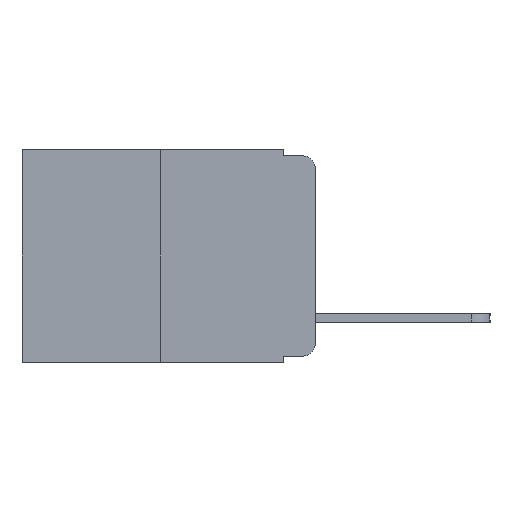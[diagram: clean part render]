
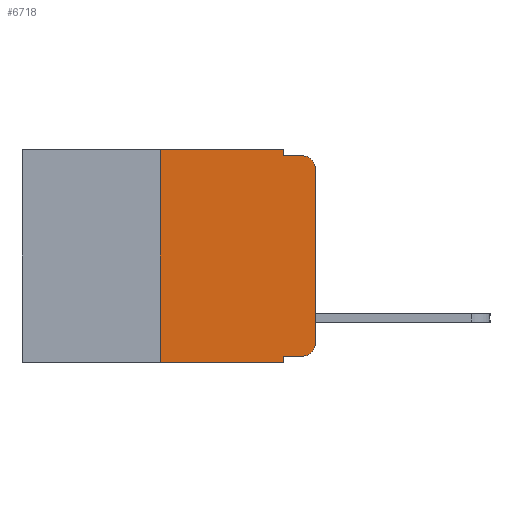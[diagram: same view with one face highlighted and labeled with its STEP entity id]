
A CAD part, left-side view. The second image highlights one B-rep face of the part: STEP entity #6718.
In plain terms, the highlighted planar face has unit normal (-1, 0, 0).
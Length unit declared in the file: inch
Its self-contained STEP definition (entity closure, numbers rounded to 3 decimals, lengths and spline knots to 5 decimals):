
#108 = EDGE_CURVE ( 'NONE', #347, #9766, #10966, .T. ) ;
#344 = LINE ( 'NONE', #10707, #2691 ) ;
#347 = VERTEX_POINT ( 'NONE', #3068 ) ;
#433 = ORIENTED_EDGE ( 'NONE', *, *, #10182, .T. ) ;
#492 = LINE ( 'NONE', #6207, #7602 ) ;
#597 = CARTESIAN_POINT ( 'NONE',  ( 0., 0.051, -0.343 ) ) ;
#741 = ORIENTED_EDGE ( 'NONE', *, *, #4778, .F. ) ;
#763 = VERTEX_POINT ( 'NONE', #1456 ) ;
#1041 = EDGE_LOOP ( 'NONE', ( #3531, #6307, #741, #2929, #4317, #3243, #433, #4896, #4964, #11048 ) ) ;
#1456 = CARTESIAN_POINT ( 'NONE',  ( 0., 0.25, 0. ) ) ;
#1543 = EDGE_CURVE ( 'NONE', #8922, #763, #7137, .T. ) ;
#1604 = VECTOR ( 'NONE', #5992, 39.37008 ) ;
#1608 = EDGE_CURVE ( 'NONE', #6167, #1844, #5993, .T. ) ;
#1651 = EDGE_CURVE ( 'NONE', #6167, #8879, #492, .T. ) ;
#1710 = EDGE_CURVE ( 'NONE', #8879, #10385, #4949, .T. ) ;
#1844 = VERTEX_POINT ( 'NONE', #597 ) ;
#1911 = CARTESIAN_POINT ( 'NONE',  ( 0., 0.473, 0. ) ) ;
#2230 = VECTOR ( 'NONE', #9896, 39.37008 ) ;
#2691 = VECTOR ( 'NONE', #4604, 39.37008 ) ;
#2699 = DIRECTION ( 'NONE',  ( 0., 0., 1. ) ) ;
#2929 = ORIENTED_EDGE ( 'NONE', *, *, #108, .F. ) ;
#3068 = CARTESIAN_POINT ( 'NONE',  ( 0., 0.051, 0. ) ) ;
#3088 = VECTOR ( 'NONE', #8854, 39.37008 ) ;
#3243 = ORIENTED_EDGE ( 'NONE', *, *, #1543, .F. ) ;
#3495 = LINE ( 'NONE', #4232, #5549 ) ;
#3531 = ORIENTED_EDGE ( 'NONE', *, *, #3992, .T. ) ;
#3609 = VERTEX_POINT ( 'NONE', #5824 ) ;
#3943 = DIRECTION ( 'NONE',  ( -1., 0., 0. ) ) ;
#3964 = CARTESIAN_POINT ( 'NONE',  ( 0., 0.02, -0.313 ) ) ;
#3992 = EDGE_CURVE ( 'NONE', #10385, #3609, #6940, .T. ) ;
#4232 = CARTESIAN_POINT ( 'NONE',  ( 0., 0.051, -0.01 ) ) ;
#4317 = ORIENTED_EDGE ( 'NONE', *, *, #7334, .F. ) ;
#4354 = CARTESIAN_POINT ( 'NONE',  ( 0., 0.051, 0. ) ) ;
#4382 = EDGE_CURVE ( 'NONE', #3609, #9949, #10866, .T. ) ;
#4604 = DIRECTION ( 'NONE',  ( 0., -1., 0. ) ) ;
#4610 = DIRECTION ( 'NONE',  ( -1., 0., 0. ) ) ;
#4635 = CARTESIAN_POINT ( 'NONE',  ( 0., 0.02, -0.03 ) ) ;
#4778 = EDGE_CURVE ( 'NONE', #9766, #9949, #3495, .T. ) ;
#4896 = ORIENTED_EDGE ( 'NONE', *, *, #1608, .F. ) ;
#4949 = CIRCLE ( 'NONE', #5562, 0.02 ) ;
#4964 = ORIENTED_EDGE ( 'NONE', *, *, #1651, .T. ) ;
#5166 = CARTESIAN_POINT ( 'NONE',  ( 0., 0.25, 0. ) ) ;
#5179 = CARTESIAN_POINT ( 'NONE',  ( 0., 0.02, -0.01 ) ) ;
#5362 = DIRECTION ( 'NONE',  ( 0., 0., -1. ) ) ;
#5549 = VECTOR ( 'NONE', #6729, 39.37008 ) ;
#5562 = AXIS2_PLACEMENT_3D ( 'NONE', #3964, #3943, #10458 ) ;
#5824 = CARTESIAN_POINT ( 'NONE',  ( 0., 0., -0.03 ) ) ;
#5992 = DIRECTION ( 'NONE',  ( 0., 0., -1. ) ) ;
#5993 = LINE ( 'NONE', #10752, #10439 ) ;
#6052 = CARTESIAN_POINT ( 'NONE',  ( 0., 0.473, 0. ) ) ;
#6167 = VERTEX_POINT ( 'NONE', #8974 ) ;
#6207 = CARTESIAN_POINT ( 'NONE',  ( 0., 0.051, -0.333 ) ) ;
#6307 = ORIENTED_EDGE ( 'NONE', *, *, #4382, .T. ) ;
#6631 = CARTESIAN_POINT ( 'NONE',  ( 0., 0., -0.313 ) ) ;
#6718 = ADVANCED_FACE ( 'NONE', ( #9049 ), #11382, .F. ) ;
#6729 = DIRECTION ( 'NONE',  ( 0., -1., 0. ) ) ;
#6940 = LINE ( 'NONE', #9470, #2230 ) ;
#7137 = LINE ( 'NONE', #5166, #9520 ) ;
#7334 = EDGE_CURVE ( 'NONE', #763, #347, #7851, .T. ) ;
#7416 = CARTESIAN_POINT ( 'NONE',  ( 0., 0.02, -0.333 ) ) ;
#7602 = VECTOR ( 'NONE', #10845, 39.37008 ) ;
#7660 = CARTESIAN_POINT ( 'NONE',  ( 0., 0.051, -0.01 ) ) ;
#7716 = AXIS2_PLACEMENT_3D ( 'NONE', #4635, #4610, #5362 ) ;
#7851 = LINE ( 'NONE', #1911, #3088 ) ;
#8854 = DIRECTION ( 'NONE',  ( 0., -1., 0. ) ) ;
#8879 = VERTEX_POINT ( 'NONE', #7416 ) ;
#8922 = VERTEX_POINT ( 'NONE', #11595 ) ;
#8974 = CARTESIAN_POINT ( 'NONE',  ( 0., 0.051, -0.333 ) ) ;
#9049 = FACE_OUTER_BOUND ( 'NONE', #1041, .T. ) ;
#9470 = CARTESIAN_POINT ( 'NONE',  ( 0., 0., 0. ) ) ;
#9520 = VECTOR ( 'NONE', #2699, 39.37008 ) ;
#9766 = VERTEX_POINT ( 'NONE', #7660 ) ;
#9896 = DIRECTION ( 'NONE',  ( 0., 0., 1. ) ) ;
#9949 = VERTEX_POINT ( 'NONE', #5179 ) ;
#10182 = EDGE_CURVE ( 'NONE', #8922, #1844, #344, .T. ) ;
#10263 = AXIS2_PLACEMENT_3D ( 'NONE', #6052, #11454, #11441 ) ;
#10385 = VERTEX_POINT ( 'NONE', #6631 ) ;
#10439 = VECTOR ( 'NONE', #11308, 39.37008 ) ;
#10458 = DIRECTION ( 'NONE',  ( 0., 0., -1. ) ) ;
#10707 = CARTESIAN_POINT ( 'NONE',  ( 0., 0.473, -0.343 ) ) ;
#10752 = CARTESIAN_POINT ( 'NONE',  ( 0., 0.051, 0. ) ) ;
#10845 = DIRECTION ( 'NONE',  ( 0., -1., 0. ) ) ;
#10866 = CIRCLE ( 'NONE', #7716, 0.02 ) ;
#10966 = LINE ( 'NONE', #4354, #1604 ) ;
#11048 = ORIENTED_EDGE ( 'NONE', *, *, #1710, .T. ) ;
#11308 = DIRECTION ( 'NONE',  ( 0., 0., -1. ) ) ;
#11382 = PLANE ( 'NONE',  #10263 ) ;
#11441 = DIRECTION ( 'NONE',  ( 0., 0., -1. ) ) ;
#11454 = DIRECTION ( 'NONE',  ( 1., 0., 0. ) ) ;
#11595 = CARTESIAN_POINT ( 'NONE',  ( 0., 0.25, -0.343 ) ) ;
